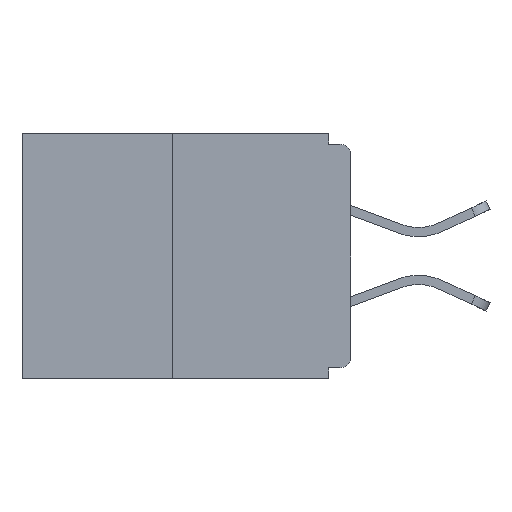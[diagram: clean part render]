
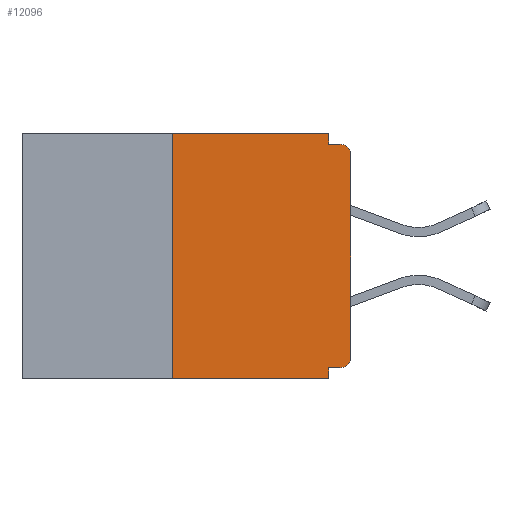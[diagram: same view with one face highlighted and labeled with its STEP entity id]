
A CAD part, left-side view. The second image highlights one B-rep face of the part: STEP entity #12096.
In plain terms, the highlighted planar face has unit normal (-1, 0, 0).
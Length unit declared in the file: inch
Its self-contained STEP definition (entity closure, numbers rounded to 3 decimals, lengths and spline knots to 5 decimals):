
#162 = DIRECTION ( 'NONE',  ( 0., 0., -1. ) ) ;
#383 = CARTESIAN_POINT ( 'NONE',  ( 0., 0.031, -0.328 ) ) ;
#558 = VECTOR ( 'NONE', #15114, 39.37008 ) ;
#564 = VECTOR ( 'NONE', #1790, 39.37008 ) ;
#719 = EDGE_CURVE ( 'NONE', #6612, #2630, #10470, .T. ) ;
#946 = CARTESIAN_POINT ( 'NONE',  ( 0., 0.015, -0.03 ) ) ;
#1191 = CARTESIAN_POINT ( 'NONE',  ( 0., 0.46, 0. ) ) ;
#1366 = LINE ( 'NONE', #7578, #13249 ) ;
#1566 = DIRECTION ( 'NONE',  ( 0., 0., 1. ) ) ;
#1790 = DIRECTION ( 'NONE',  ( 0., 0., 1. ) ) ;
#1911 = CARTESIAN_POINT ( 'NONE',  ( 0., 0., -0.328 ) ) ;
#2014 = EDGE_CURVE ( 'NONE', #10706, #2436, #2381, .T. ) ;
#2381 = LINE ( 'NONE', #9479, #3975 ) ;
#2436 = VERTEX_POINT ( 'NONE', #2804 ) ;
#2547 = EDGE_CURVE ( 'NONE', #11901, #6612, #6972, .T. ) ;
#2630 = VERTEX_POINT ( 'NONE', #17045 ) ;
#2804 = CARTESIAN_POINT ( 'NONE',  ( 0., 0.031, 0. ) ) ;
#3215 = CARTESIAN_POINT ( 'NONE',  ( 0., 0., -0.313 ) ) ;
#3461 = ORIENTED_EDGE ( 'NONE', *, *, #3901, .T. ) ;
#3901 = EDGE_CURVE ( 'NONE', #5833, #8545, #10607, .T. ) ;
#3975 = VECTOR ( 'NONE', #5020, 39.37008 ) ;
#4073 = ORIENTED_EDGE ( 'NONE', *, *, #6154, .F. ) ;
#4343 = ORIENTED_EDGE ( 'NONE', *, *, #16321, .T. ) ;
#4374 = ORIENTED_EDGE ( 'NONE', *, *, #14723, .T. ) ;
#4579 = ORIENTED_EDGE ( 'NONE', *, *, #14421, .T. ) ;
#5020 = DIRECTION ( 'NONE',  ( 0., -1., 0. ) ) ;
#5115 = DIRECTION ( 'NONE',  ( -1., 0., 0. ) ) ;
#5199 = CARTESIAN_POINT ( 'NONE',  ( 0., 0., -0.03 ) ) ;
#5381 = CARTESIAN_POINT ( 'NONE',  ( 0., 0.25, 0. ) ) ;
#5638 = CARTESIAN_POINT ( 'NONE',  ( 0., 0.25, -0.343 ) ) ;
#5833 = VERTEX_POINT ( 'NONE', #3215 ) ;
#5981 = DIRECTION ( 'NONE',  ( 0., -1., 0. ) ) ;
#6154 = EDGE_CURVE ( 'NONE', #15201, #11755, #1366, .T. ) ;
#6202 = CIRCLE ( 'NONE', #6352, 0.015 ) ;
#6232 = CARTESIAN_POINT ( 'NONE',  ( 0., 0.031, -0.343 ) ) ;
#6352 = AXIS2_PLACEMENT_3D ( 'NONE', #946, #5115, #11173 ) ;
#6558 = DIRECTION ( 'NONE',  ( 0., 0., -1. ) ) ;
#6612 = VERTEX_POINT ( 'NONE', #383 ) ;
#6972 = LINE ( 'NONE', #1911, #558 ) ;
#7038 = VECTOR ( 'NONE', #1566, 39.37008 ) ;
#7044 = LINE ( 'NONE', #15226, #8225 ) ;
#7087 = DIRECTION ( 'NONE',  ( 1., 0., 0. ) ) ;
#7355 = CARTESIAN_POINT ( 'NONE',  ( 0., 0.25, 0. ) ) ;
#7578 = CARTESIAN_POINT ( 'NONE',  ( 0., 0., -0.015 ) ) ;
#7580 = DIRECTION ( 'NONE',  ( 0., 0., -1. ) ) ;
#8225 = VECTOR ( 'NONE', #14950, 39.37008 ) ;
#8532 = EDGE_LOOP ( 'NONE', ( #16425, #10417, #4343, #18707, #12869, #4579, #3461, #4374, #4073, #18557 ) ) ;
#8545 = VERTEX_POINT ( 'NONE', #5199 ) ;
#9479 = CARTESIAN_POINT ( 'NONE',  ( 0., 0.46, 0. ) ) ;
#10188 = DIRECTION ( 'NONE',  ( 0., -1., 0. ) ) ;
#10366 = AXIS2_PLACEMENT_3D ( 'NONE', #13884, #16871, #6558 ) ;
#10417 = ORIENTED_EDGE ( 'NONE', *, *, #10937, .F. ) ;
#10470 = LINE ( 'NONE', #6232, #14581 ) ;
#10607 = LINE ( 'NONE', #14915, #564 ) ;
#10706 = VERTEX_POINT ( 'NONE', #5381 ) ;
#10937 = EDGE_CURVE ( 'NONE', #18921, #10706, #14819, .T. ) ;
#11173 = DIRECTION ( 'NONE',  ( 0., 0., -1. ) ) ;
#11219 = LINE ( 'NONE', #12974, #11661 ) ;
#11661 = VECTOR ( 'NONE', #10188, 39.37008 ) ;
#11755 = VERTEX_POINT ( 'NONE', #12686 ) ;
#11901 = VERTEX_POINT ( 'NONE', #14902 ) ;
#12096 = ADVANCED_FACE ( 'NONE', ( #17514 ), #14436, .F. ) ;
#12686 = CARTESIAN_POINT ( 'NONE',  ( 0., 0.015, -0.015 ) ) ;
#12869 = ORIENTED_EDGE ( 'NONE', *, *, #2547, .F. ) ;
#12974 = CARTESIAN_POINT ( 'NONE',  ( 0., 0.46, -0.343 ) ) ;
#13249 = VECTOR ( 'NONE', #5981, 39.37008 ) ;
#13790 = AXIS2_PLACEMENT_3D ( 'NONE', #1191, #7087, #162 ) ;
#13884 = CARTESIAN_POINT ( 'NONE',  ( 0., 0.015, -0.313 ) ) ;
#14421 = EDGE_CURVE ( 'NONE', #11901, #5833, #16537, .T. ) ;
#14436 = PLANE ( 'NONE',  #13790 ) ;
#14581 = VECTOR ( 'NONE', #7580, 39.37008 ) ;
#14723 = EDGE_CURVE ( 'NONE', #8545, #11755, #6202, .T. ) ;
#14819 = LINE ( 'NONE', #7355, #7038 ) ;
#14902 = CARTESIAN_POINT ( 'NONE',  ( 0., 0.015, -0.328 ) ) ;
#14915 = CARTESIAN_POINT ( 'NONE',  ( 0., 0., 0. ) ) ;
#14950 = DIRECTION ( 'NONE',  ( 0., 0., -1. ) ) ;
#15114 = DIRECTION ( 'NONE',  ( 0., 1., 0. ) ) ;
#15201 = VERTEX_POINT ( 'NONE', #17770 ) ;
#15226 = CARTESIAN_POINT ( 'NONE',  ( 0., 0.031, 0. ) ) ;
#16321 = EDGE_CURVE ( 'NONE', #18921, #2630, #11219, .T. ) ;
#16425 = ORIENTED_EDGE ( 'NONE', *, *, #2014, .F. ) ;
#16537 = CIRCLE ( 'NONE', #10366, 0.015 ) ;
#16871 = DIRECTION ( 'NONE',  ( -1., 0., 0. ) ) ;
#17045 = CARTESIAN_POINT ( 'NONE',  ( 0., 0.031, -0.343 ) ) ;
#17514 = FACE_OUTER_BOUND ( 'NONE', #8532, .T. ) ;
#17770 = CARTESIAN_POINT ( 'NONE',  ( 0., 0.031, -0.015 ) ) ;
#18027 = EDGE_CURVE ( 'NONE', #2436, #15201, #7044, .T. ) ;
#18557 = ORIENTED_EDGE ( 'NONE', *, *, #18027, .F. ) ;
#18707 = ORIENTED_EDGE ( 'NONE', *, *, #719, .F. ) ;
#18921 = VERTEX_POINT ( 'NONE', #5638 ) ;
